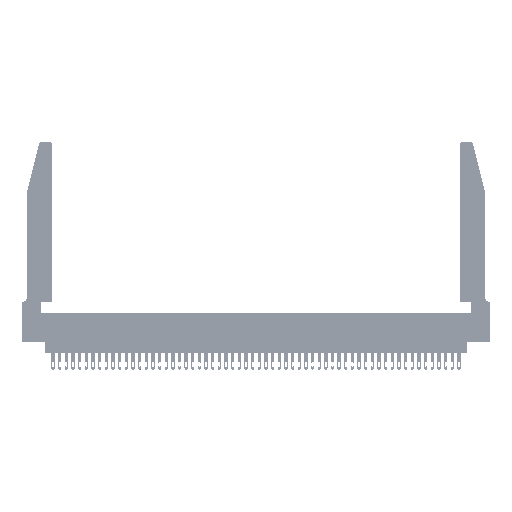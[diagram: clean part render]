
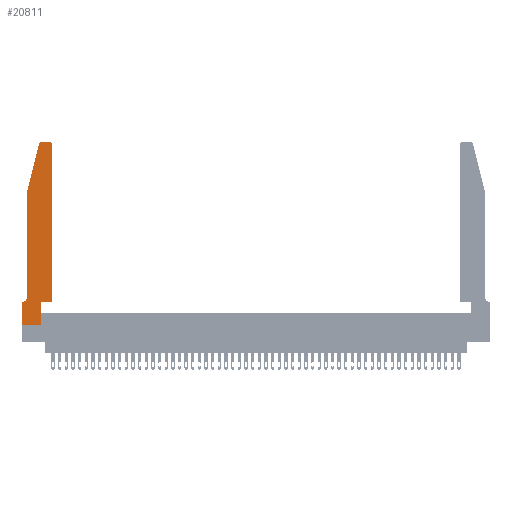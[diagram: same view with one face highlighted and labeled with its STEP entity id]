
A CAD part, top view. The second image highlights one B-rep face of the part: STEP entity #20811.
In plain terms, the highlighted planar face has unit normal (0, 0, 1).
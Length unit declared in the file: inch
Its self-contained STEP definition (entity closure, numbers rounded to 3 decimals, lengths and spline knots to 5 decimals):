
#1046 = DIRECTION ( 'NONE',  ( 0., 1., 0. ) ) ;
#1115 = CARTESIAN_POINT ( 'NONE',  ( 0.4205, 2.75, 0.37 ) ) ;
#2166 = VERTEX_POINT ( 'NONE', #13068 ) ;
#3009 = CIRCLE ( 'NONE', #44371, 0.03 ) ;
#3416 = AXIS2_PLACEMENT_3D ( 'NONE', #6278, #22368, #30219 ) ;
#3679 = LINE ( 'NONE', #39796, #46697 ) ;
#3710 = EDGE_CURVE ( 'NONE', #28003, #47642, #3009, .T. ) ;
#3988 = VECTOR ( 'NONE', #22570, 39.37008 ) ;
#5350 = CARTESIAN_POINT ( 'NONE',  ( 0.284, 2.72, 0.37 ) ) ;
#6278 = CARTESIAN_POINT ( 'NONE',  ( 0.0055, 0.42, 0.37 ) ) ;
#6849 = ORIENTED_EDGE ( 'NONE', *, *, #36637, .T. ) ;
#7065 = CARTESIAN_POINT ( 'NONE',  ( 0., 0., 0.37 ) ) ;
#7678 = AXIS2_PLACEMENT_3D ( 'NONE', #37438, #13563, #13734 ) ;
#8082 = FACE_OUTER_BOUND ( 'NONE', #16414, .T. ) ;
#8253 = VERTEX_POINT ( 'NONE', #44519 ) ;
#8517 = ORIENTED_EDGE ( 'NONE', *, *, #35524, .T. ) ;
#8702 = EDGE_CURVE ( 'NONE', #39783, #8253, #31067, .T. ) ;
#8764 = CARTESIAN_POINT ( 'NONE',  ( 0.0755, 2., 0.37 ) ) ;
#9704 = EDGE_CURVE ( 'NONE', #2166, #44734, #15574, .T. ) ;
#9996 = DIRECTION ( 'NONE',  ( -1., 0., 0. ) ) ;
#10816 = CARTESIAN_POINT ( 'NONE',  ( 0., 0., 0.37 ) ) ;
#12434 = ORIENTED_EDGE ( 'NONE', *, *, #47112, .T. ) ;
#12995 = VERTEX_POINT ( 'NONE', #7065 ) ;
#13068 = CARTESIAN_POINT ( 'NONE',  ( 0.0055, 0.35, 0.37 ) ) ;
#13563 = DIRECTION ( 'NONE',  ( 0., 0., 1. ) ) ;
#13734 = DIRECTION ( 'NONE',  ( 1., 0., 0. ) ) ;
#14161 = LINE ( 'NONE', #40646, #43115 ) ;
#15470 = ORIENTED_EDGE ( 'NONE', *, *, #17973, .T. ) ;
#15574 = LINE ( 'NONE', #24953, #35816 ) ;
#16270 = ORIENTED_EDGE ( 'NONE', *, *, #26289, .T. ) ;
#16412 = ORIENTED_EDGE ( 'NONE', *, *, #9704, .T. ) ;
#16414 = EDGE_LOOP ( 'NONE', ( #16270, #50714, #45645, #34520, #8517, #16412, #18832, #15470, #20672, #6849, #12434, #46363 ) ) ;
#16434 = DIRECTION ( 'NONE',  ( -0.239, -0.971, 0. ) ) ;
#17269 = DIRECTION ( 'NONE',  ( 1., 0., 0. ) ) ;
#17973 = EDGE_CURVE ( 'NONE', #12995, #41148, #27478, .T. ) ;
#18239 = CARTESIAN_POINT ( 'NONE',  ( 0.2605, 2.75, 0.37 ) ) ;
#18832 = ORIENTED_EDGE ( 'NONE', *, *, #43279, .T. ) ;
#19205 = CARTESIAN_POINT ( 'NONE',  ( 0.4505, 0.35, 0.37 ) ) ;
#19571 = VECTOR ( 'NONE', #16434, 39.37008 ) ;
#19807 = DIRECTION ( 'NONE',  ( 1., 0., 0. ) ) ;
#20672 = ORIENTED_EDGE ( 'NONE', *, *, #32971, .T. ) ;
#20811 = ADVANCED_FACE ( 'NONE', ( #8082 ), #38086, .T. ) ;
#22368 = DIRECTION ( 'NONE',  ( 0., 0., -1. ) ) ;
#22570 = DIRECTION ( 'NONE',  ( 0., 1., 0. ) ) ;
#23032 = CARTESIAN_POINT ( 'NONE',  ( 0., 0., 0.37 ) ) ;
#23108 = VECTOR ( 'NONE', #42359, 39.37008 ) ;
#23193 = DIRECTION ( 'NONE',  ( 0., -1., 0. ) ) ;
#23691 = CARTESIAN_POINT ( 'NONE',  ( 0.2865, 0., 0.37 ) ) ;
#24553 = LINE ( 'NONE', #23032, #33734 ) ;
#24953 = CARTESIAN_POINT ( 'NONE',  ( 0.0755, 0.35, 0.37 ) ) ;
#25159 = VERTEX_POINT ( 'NONE', #19205 ) ;
#26067 = LINE ( 'NONE', #49370, #3988 ) ;
#26289 = EDGE_CURVE ( 'NONE', #47549, #28003, #38281, .T. ) ;
#26621 = DIRECTION ( 'NONE',  ( 0., 0., 1. ) ) ;
#26898 = CARTESIAN_POINT ( 'NONE',  ( 0.0755, 2., 0.37 ) ) ;
#27478 = LINE ( 'NONE', #10816, #47152 ) ;
#28003 = VERTEX_POINT ( 'NONE', #28150 ) ;
#28150 = CARTESIAN_POINT ( 'NONE',  ( 0.284, 2.75, 0.37 ) ) ;
#29350 = DIRECTION ( 'NONE',  ( 0., 0., 1. ) ) ;
#29675 = AXIS2_PLACEMENT_3D ( 'NONE', #50143, #26621, #34150 ) ;
#30056 = LINE ( 'NONE', #8764, #19571 ) ;
#30133 = CARTESIAN_POINT ( 'NONE',  ( 0.4505, 2.72, 0.37 ) ) ;
#30179 = CARTESIAN_POINT ( 'NONE',  ( 0.2865, 0.35, 0.37 ) ) ;
#30219 = DIRECTION ( 'NONE',  ( -1., 0., 0. ) ) ;
#30685 = VERTEX_POINT ( 'NONE', #30179 ) ;
#31067 = LINE ( 'NONE', #26898, #23108 ) ;
#32014 = CARTESIAN_POINT ( 'NONE',  ( 0.0755, 2., 0.37 ) ) ;
#32468 = CARTESIAN_POINT ( 'NONE',  ( 0., 0.35, 0.37 ) ) ;
#32971 = EDGE_CURVE ( 'NONE', #41148, #30685, #14161, .T. ) ;
#33734 = VECTOR ( 'NONE', #23193, 39.37008 ) ;
#33888 = EDGE_CURVE ( 'NONE', #47642, #39783, #30056, .T. ) ;
#34150 = DIRECTION ( 'NONE',  ( 1., 0., 0. ) ) ;
#34520 = ORIENTED_EDGE ( 'NONE', *, *, #8702, .T. ) ;
#35344 = EDGE_CURVE ( 'NONE', #41583, #47549, #41282, .T. ) ;
#35524 = EDGE_CURVE ( 'NONE', #8253, #2166, #48062, .T. ) ;
#35816 = VECTOR ( 'NONE', #9996, 39.37008 ) ;
#36446 = VECTOR ( 'NONE', #46308, 39.37008 ) ;
#36637 = EDGE_CURVE ( 'NONE', #30685, #25159, #3679, .T. ) ;
#37438 = CARTESIAN_POINT ( 'NONE',  ( 0.4205, 2.72, 0.37 ) ) ;
#38086 = PLANE ( 'NONE',  #29675 ) ;
#38281 = LINE ( 'NONE', #18239, #36446 ) ;
#39783 = VERTEX_POINT ( 'NONE', #32014 ) ;
#39796 = CARTESIAN_POINT ( 'NONE',  ( 0.4505, 0.35, 0.37 ) ) ;
#40554 = CARTESIAN_POINT ( 'NONE',  ( 0.25487, 2.72718, 0.37 ) ) ;
#40646 = CARTESIAN_POINT ( 'NONE',  ( 0.2865, 0.35, 0.37 ) ) ;
#41148 = VERTEX_POINT ( 'NONE', #23691 ) ;
#41282 = CIRCLE ( 'NONE', #7678, 0.03 ) ;
#41583 = VERTEX_POINT ( 'NONE', #30133 ) ;
#42359 = DIRECTION ( 'NONE',  ( 0., -1., 0. ) ) ;
#43115 = VECTOR ( 'NONE', #1046, 39.37008 ) ;
#43279 = EDGE_CURVE ( 'NONE', #44734, #12995, #24553, .T. ) ;
#44371 = AXIS2_PLACEMENT_3D ( 'NONE', #5350, #29350, #17269 ) ;
#44519 = CARTESIAN_POINT ( 'NONE',  ( 0.0755, 0.42, 0.37 ) ) ;
#44734 = VERTEX_POINT ( 'NONE', #32468 ) ;
#45645 = ORIENTED_EDGE ( 'NONE', *, *, #33888, .T. ) ;
#46226 = DIRECTION ( 'NONE',  ( 1., 0., 0. ) ) ;
#46308 = DIRECTION ( 'NONE',  ( -1., 0., 0. ) ) ;
#46363 = ORIENTED_EDGE ( 'NONE', *, *, #35344, .T. ) ;
#46697 = VECTOR ( 'NONE', #19807, 39.37008 ) ;
#47112 = EDGE_CURVE ( 'NONE', #25159, #41583, #26067, .T. ) ;
#47152 = VECTOR ( 'NONE', #46226, 39.37008 ) ;
#47549 = VERTEX_POINT ( 'NONE', #1115 ) ;
#47642 = VERTEX_POINT ( 'NONE', #40554 ) ;
#48062 = CIRCLE ( 'NONE', #3416, 0.07 ) ;
#49370 = CARTESIAN_POINT ( 'NONE',  ( 0.4505, 0.35, 0.37 ) ) ;
#50143 = CARTESIAN_POINT ( 'NONE',  ( 0., 0.35, 0.37 ) ) ;
#50714 = ORIENTED_EDGE ( 'NONE', *, *, #3710, .T. ) ;
